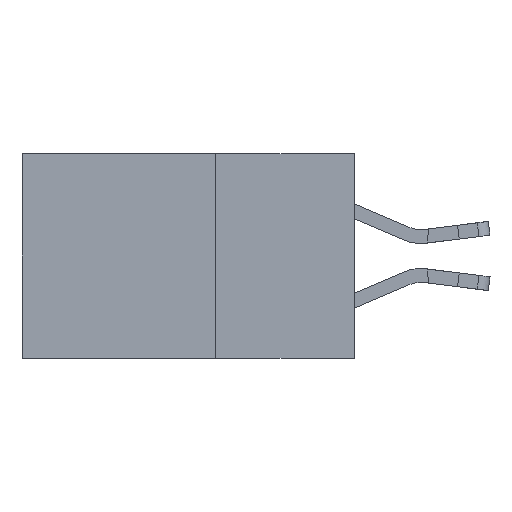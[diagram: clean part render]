
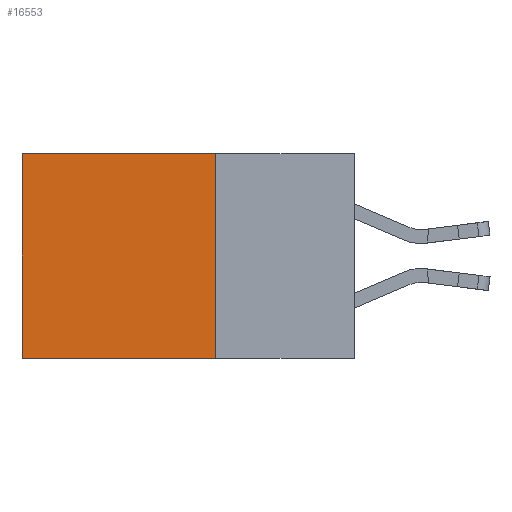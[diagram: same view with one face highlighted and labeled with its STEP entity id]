
A CAD part, left-side view. The second image highlights one B-rep face of the part: STEP entity #16553.
In plain terms, the highlighted planar face has unit normal (-1, 0, 0).
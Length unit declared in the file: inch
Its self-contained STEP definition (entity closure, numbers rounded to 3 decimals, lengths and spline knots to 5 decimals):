
#184 = CARTESIAN_POINT ( 'NONE',  ( 0.298, 0.6, 0. ) ) ;
#210 = LINE ( 'NONE', #20125, #4911 ) ;
#417 = CARTESIAN_POINT ( 'NONE',  ( 0.298, 0.6, 0. ) ) ;
#1277 = CARTESIAN_POINT ( 'NONE',  ( 0.298, 0.25, 0. ) ) ;
#1509 = LINE ( 'NONE', #15660, #7433 ) ;
#2260 = VECTOR ( 'NONE', #11686, 39.37008 ) ;
#2532 = LINE ( 'NONE', #417, #13748 ) ;
#3034 = VERTEX_POINT ( 'NONE', #184 ) ;
#3716 = EDGE_CURVE ( 'NONE', #3034, #5026, #2532, .T. ) ;
#3769 = ORIENTED_EDGE ( 'NONE', *, *, #17787, .F. ) ;
#4307 = DIRECTION ( 'NONE',  ( 1., 0., 0. ) ) ;
#4347 = DIRECTION ( 'NONE',  ( 0., 1., 0. ) ) ;
#4911 = VECTOR ( 'NONE', #11421, 39.37008 ) ;
#5026 = VERTEX_POINT ( 'NONE', #11490 ) ;
#5583 = AXIS2_PLACEMENT_3D ( 'NONE', #1277, #4307, #15461 ) ;
#7245 = ORIENTED_EDGE ( 'NONE', *, *, #3716, .T. ) ;
#7433 = VECTOR ( 'NONE', #4347, 39.37008 ) ;
#7812 = VERTEX_POINT ( 'NONE', #11606 ) ;
#10508 = CARTESIAN_POINT ( 'NONE',  ( 0.298, 0.25, 0. ) ) ;
#11131 = VERTEX_POINT ( 'NONE', #10508 ) ;
#11421 = DIRECTION ( 'NONE',  ( 0., 1., 0. ) ) ;
#11490 = CARTESIAN_POINT ( 'NONE',  ( 0.298, 0.6, -0.37 ) ) ;
#11606 = CARTESIAN_POINT ( 'NONE',  ( 0.298, 0.25, -0.37 ) ) ;
#11686 = DIRECTION ( 'NONE',  ( 0., 0., -1. ) ) ;
#13165 = DIRECTION ( 'NONE',  ( 0., 0., -1. ) ) ;
#13748 = VECTOR ( 'NONE', #13165, 39.37008 ) ;
#14740 = EDGE_CURVE ( 'NONE', #7812, #5026, #210, .T. ) ;
#15461 = DIRECTION ( 'NONE',  ( 0., 0., -1. ) ) ;
#15607 = EDGE_LOOP ( 'NONE', ( #7245, #15754, #3769, #17205 ) ) ;
#15660 = CARTESIAN_POINT ( 'NONE',  ( 0.298, 0.25, 0. ) ) ;
#15754 = ORIENTED_EDGE ( 'NONE', *, *, #14740, .F. ) ;
#16553 = ADVANCED_FACE ( 'NONE', ( #16865 ), #20404, .F. ) ;
#16865 = FACE_OUTER_BOUND ( 'NONE', #15607, .T. ) ;
#17205 = ORIENTED_EDGE ( 'NONE', *, *, #18432, .T. ) ;
#17787 = EDGE_CURVE ( 'NONE', #11131, #7812, #20207, .T. ) ;
#18432 = EDGE_CURVE ( 'NONE', #11131, #3034, #1509, .T. ) ;
#19640 = CARTESIAN_POINT ( 'NONE',  ( 0.298, 0.25, 0. ) ) ;
#20125 = CARTESIAN_POINT ( 'NONE',  ( 0.298, 0.25, -0.37 ) ) ;
#20207 = LINE ( 'NONE', #19640, #2260 ) ;
#20404 = PLANE ( 'NONE',  #5583 ) ;
